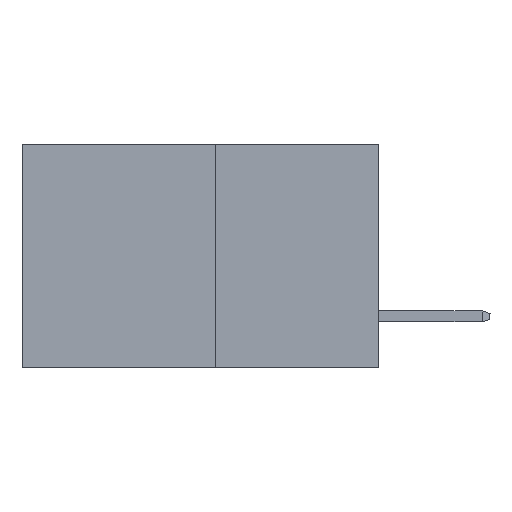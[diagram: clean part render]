
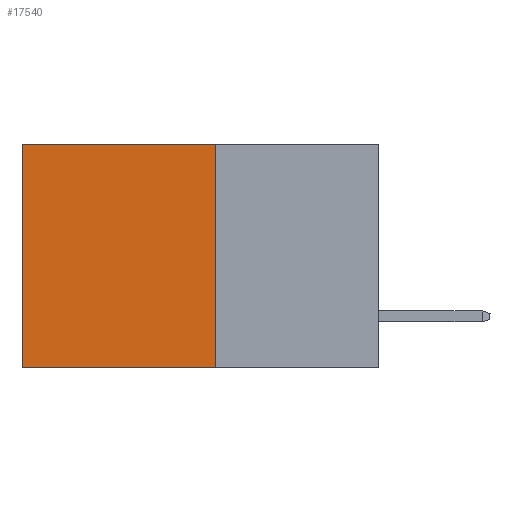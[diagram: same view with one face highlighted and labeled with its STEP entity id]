
A CAD part, left-side view. The second image highlights one B-rep face of the part: STEP entity #17540.
In plain terms, the highlighted planar face has unit normal (-1, 0, 0).
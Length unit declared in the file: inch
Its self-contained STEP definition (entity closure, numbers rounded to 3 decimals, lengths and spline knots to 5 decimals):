
#2881 = VECTOR ( 'NONE', #27803, 39.37008 ) ;
#4345 = DIRECTION ( 'NONE',  ( 1., 0., 0. ) ) ;
#4566 = CARTESIAN_POINT ( 'NONE',  ( 0.277, 0.59, -0.37 ) ) ;
#6069 = CARTESIAN_POINT ( 'NONE',  ( 0.277, 0.27, 0. ) ) ;
#6681 = VECTOR ( 'NONE', #13159, 39.37008 ) ;
#7570 = EDGE_CURVE ( 'NONE', #21164, #14812, #15707, .T. ) ;
#8365 = ORIENTED_EDGE ( 'NONE', *, *, #7570, .F. ) ;
#8970 = AXIS2_PLACEMENT_3D ( 'NONE', #14711, #4345, #22741 ) ;
#8971 = EDGE_CURVE ( 'NONE', #26637, #14812, #10624, .T. ) ;
#10510 = CARTESIAN_POINT ( 'NONE',  ( 0.277, 0.59, -0.37 ) ) ;
#10624 = LINE ( 'NONE', #4566, #23887 ) ;
#13159 = DIRECTION ( 'NONE',  ( 0., 1., 0. ) ) ;
#13648 = FACE_OUTER_BOUND ( 'NONE', #20468, .T. ) ;
#13751 = DIRECTION ( 'NONE',  ( 0., 0., -1. ) ) ;
#14711 = CARTESIAN_POINT ( 'NONE',  ( 0.277, 0.27, -0.37 ) ) ;
#14812 = VERTEX_POINT ( 'NONE', #10510 ) ;
#14839 = ORIENTED_EDGE ( 'NONE', *, *, #19069, .T. ) ;
#15707 = LINE ( 'NONE', #21565, #16556 ) ;
#16424 = CARTESIAN_POINT ( 'NONE',  ( 0.277, 0.59, 0. ) ) ;
#16556 = VECTOR ( 'NONE', #19171, 39.37008 ) ;
#17246 = ORIENTED_EDGE ( 'NONE', *, *, #20655, .F. ) ;
#17540 = ADVANCED_FACE ( 'NONE', ( #13648 ), #25267, .F. ) ;
#19069 = EDGE_CURVE ( 'NONE', #32815, #26637, #33116, .T. ) ;
#19171 = DIRECTION ( 'NONE',  ( 0., 1., 0. ) ) ;
#19356 = CARTESIAN_POINT ( 'NONE',  ( 0.277, 0.27, -0.37 ) ) ;
#20468 = EDGE_LOOP ( 'NONE', ( #31125, #8365, #17246, #14839 ) ) ;
#20655 = EDGE_CURVE ( 'NONE', #32815, #21164, #30912, .T. ) ;
#21164 = VERTEX_POINT ( 'NONE', #19356 ) ;
#21565 = CARTESIAN_POINT ( 'NONE',  ( 0.277, 0.27, -0.37 ) ) ;
#22741 = DIRECTION ( 'NONE',  ( 0., 0., -1. ) ) ;
#23887 = VECTOR ( 'NONE', #13751, 39.37008 ) ;
#25267 = PLANE ( 'NONE',  #8970 ) ;
#26637 = VERTEX_POINT ( 'NONE', #16424 ) ;
#27803 = DIRECTION ( 'NONE',  ( 0., 0., -1. ) ) ;
#29059 = CARTESIAN_POINT ( 'NONE',  ( 0.277, 0.27, 0. ) ) ;
#30377 = CARTESIAN_POINT ( 'NONE',  ( 0.277, 0.27, -0.37 ) ) ;
#30912 = LINE ( 'NONE', #30377, #2881 ) ;
#31125 = ORIENTED_EDGE ( 'NONE', *, *, #8971, .T. ) ;
#32815 = VERTEX_POINT ( 'NONE', #6069 ) ;
#33116 = LINE ( 'NONE', #29059, #6681 ) ;
